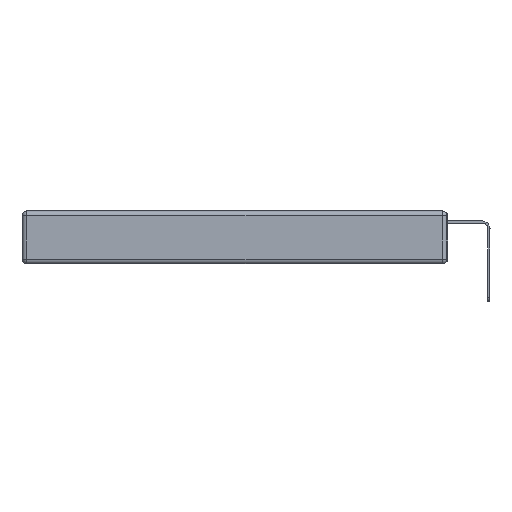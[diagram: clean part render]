
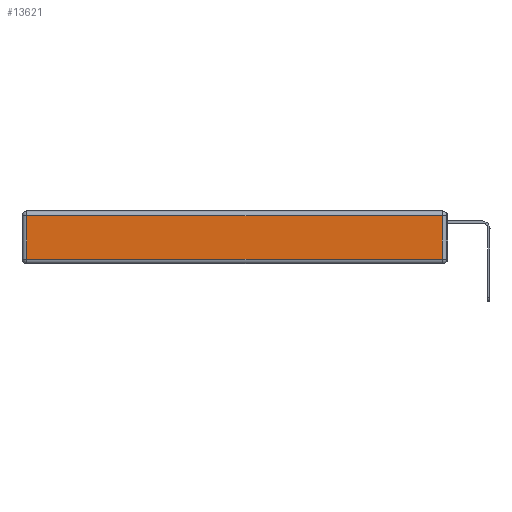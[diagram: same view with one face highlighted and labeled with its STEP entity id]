
A CAD part, left-side view. The second image highlights one B-rep face of the part: STEP entity #13621.
In plain terms, the highlighted planar face has unit normal (-1, 0, 0).
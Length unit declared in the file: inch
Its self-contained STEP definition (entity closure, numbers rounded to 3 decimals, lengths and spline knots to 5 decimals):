
#2434 = FACE_OUTER_BOUND ( 'NONE', #21016, .T. ) ;
#4389 = CARTESIAN_POINT ( 'NONE',  ( 0., 2.72, -0.313 ) ) ;
#5426 = DIRECTION ( 'NONE',  ( 0., 0., 1. ) ) ;
#6171 = CARTESIAN_POINT ( 'NONE',  ( 0., 0., -0.313 ) ) ;
#6320 = ORIENTED_EDGE ( 'NONE', *, *, #6834, .T. ) ;
#6395 = ORIENTED_EDGE ( 'NONE', *, *, #18712, .T. ) ;
#6834 = EDGE_CURVE ( 'NONE', #21433, #16637, #9168, .T. ) ;
#9120 = PLANE ( 'NONE',  #20279 ) ;
#9168 = LINE ( 'NONE', #14649, #12625 ) ;
#9281 = CARTESIAN_POINT ( 'NONE',  ( 0., 0.03, -0.313 ) ) ;
#10858 = CARTESIAN_POINT ( 'NONE',  ( 0., 2.75, -0.03 ) ) ;
#11432 = DIRECTION ( 'NONE',  ( 0., -1., 0. ) ) ;
#11747 = CARTESIAN_POINT ( 'NONE',  ( 0., 2.72, -0.03 ) ) ;
#11928 = VECTOR ( 'NONE', #11432, 39.37008 ) ;
#12195 = CARTESIAN_POINT ( 'NONE',  ( 0., 0.03, -0.343 ) ) ;
#12397 = LINE ( 'NONE', #10858, #20863 ) ;
#12625 = VECTOR ( 'NONE', #21631, 39.37008 ) ;
#12667 = LINE ( 'NONE', #12195, #17680 ) ;
#13621 = ADVANCED_FACE ( 'NONE', ( #2434 ), #9120, .T. ) ;
#13815 = ORIENTED_EDGE ( 'NONE', *, *, #18155, .T. ) ;
#14649 = CARTESIAN_POINT ( 'NONE',  ( 0., 2.72, -0.343 ) ) ;
#15836 = DIRECTION ( 'NONE',  ( 0., 0., 1. ) ) ;
#15915 = CARTESIAN_POINT ( 'NONE',  ( 0., 0., -0.343 ) ) ;
#15964 = DIRECTION ( 'NONE',  ( 0., 1., 0. ) ) ;
#16199 = VERTEX_POINT ( 'NONE', #20046 ) ;
#16395 = LINE ( 'NONE', #6171, #11928 ) ;
#16637 = VERTEX_POINT ( 'NONE', #4389 ) ;
#17646 = ORIENTED_EDGE ( 'NONE', *, *, #21237, .T. ) ;
#17680 = VECTOR ( 'NONE', #5426, 39.37008 ) ;
#18155 = EDGE_CURVE ( 'NONE', #21139, #16199, #12667, .T. ) ;
#18712 = EDGE_CURVE ( 'NONE', #16199, #21433, #12397, .T. ) ;
#19271 = DIRECTION ( 'NONE',  ( -1., 0., 0. ) ) ;
#20046 = CARTESIAN_POINT ( 'NONE',  ( 0., 0.03, -0.03 ) ) ;
#20279 = AXIS2_PLACEMENT_3D ( 'NONE', #15915, #19271, #15836 ) ;
#20863 = VECTOR ( 'NONE', #15964, 39.37008 ) ;
#21016 = EDGE_LOOP ( 'NONE', ( #17646, #13815, #6395, #6320 ) ) ;
#21139 = VERTEX_POINT ( 'NONE', #9281 ) ;
#21237 = EDGE_CURVE ( 'NONE', #16637, #21139, #16395, .T. ) ;
#21433 = VERTEX_POINT ( 'NONE', #11747 ) ;
#21631 = DIRECTION ( 'NONE',  ( 0., 0., -1. ) ) ;
